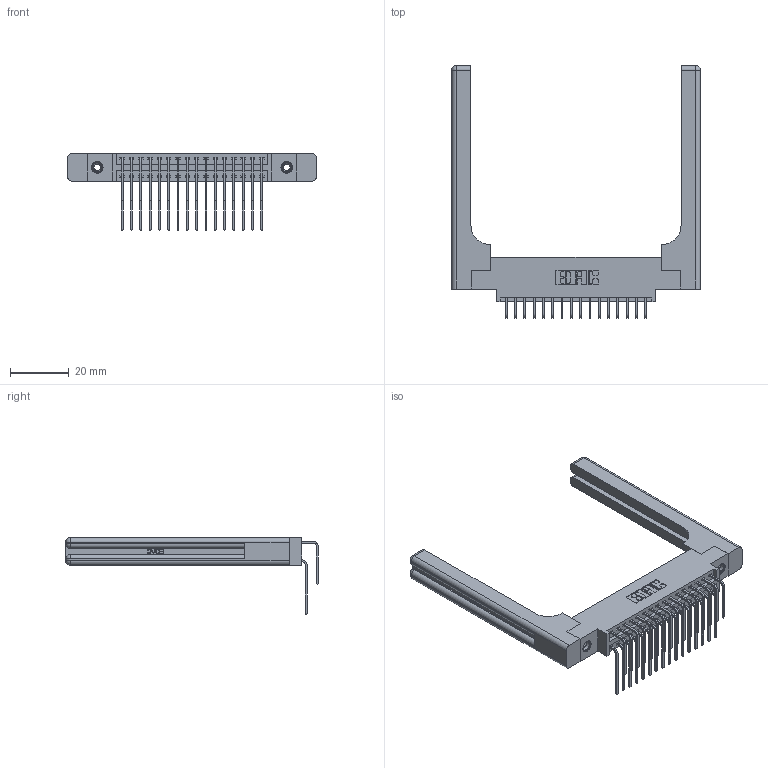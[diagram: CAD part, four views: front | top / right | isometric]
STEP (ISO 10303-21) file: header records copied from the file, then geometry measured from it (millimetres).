
FILE_DESCRIPTION (( 'STEP AP203' ), '1' );
FILE_NAME ('396-032-559-858.STEP', '2019-11-03T06:48:42', ( '' ), ( '' ), 'SwSTEP 2.0', 'SolidWorks 2016', '' );
FILE_SCHEMA (( 'CONFIG_CONTROL_DESIGN' ));
Length unit declared in the file: inch
Products named in the file (6): 396-032-559-858; 345-292-001_559 Tail - 2; 346-220-058_345-220-058; 345-292-001_558 559 Tail - 1; 346 Part_0.170 Offset - 0.156 Dia-TH; 345-250-001_345-250-001-102
Assembly tree (37 placements, depth 2):
  396-032-559-858
    346 Part_0.170 Offset - 0.156 Dia-TH
    345-292-001_558 559 Tail - 1  x16
    345-292-001_559 Tail - 2  x16
    345-250-001_345-250-001-102  x2
    346-220-058_345-220-058  x2
Bounding box: 84.86 x 86.17 x 26.16 mm (x, y, z)
Volume: 15597.3 mm3; surface area: 16767.6 mm2
Topology: 37 solids, 37 shells, 2110 faces, 6159 edges, 4042 vertices
Faces by surface type: plane 1412, cylinder 638, bspline 36, cone 12, sphere 8, torus 4
Entity records: 21040 total; most frequent: CARTESIAN_POINT 4564, ORIENTED_EDGE 3244, DIRECTION 2978, EDGE_CURVE 1622, VECTOR 1294, LINE 1294, VERTEX_POINT 1070, AXIS2_PLACEMENT_3D 842
